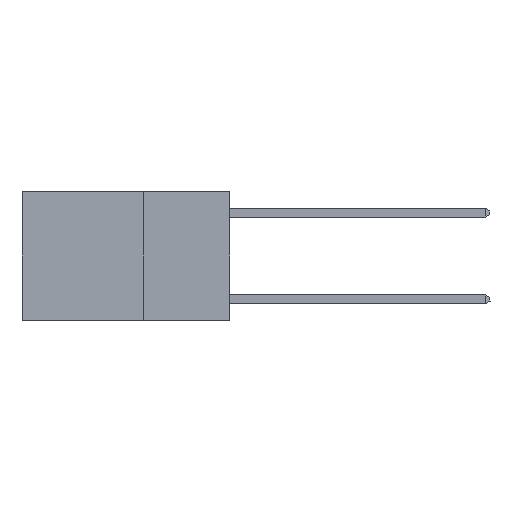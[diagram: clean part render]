
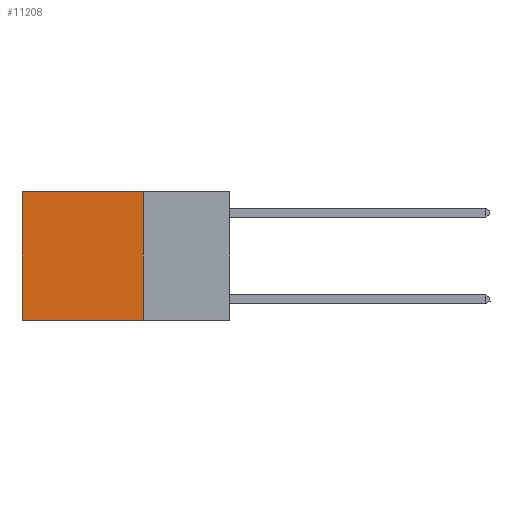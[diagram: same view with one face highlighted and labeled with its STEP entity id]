
A CAD part, left-side view. The second image highlights one B-rep face of the part: STEP entity #11208.
In plain terms, the highlighted planar face has unit normal (-1, 0, 0).
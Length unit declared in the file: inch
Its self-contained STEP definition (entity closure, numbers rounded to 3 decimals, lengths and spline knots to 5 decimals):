
#1647 = CARTESIAN_POINT ( 'NONE',  ( 0.2625, 0.25, -0.37 ) ) ;
#2229 = VECTOR ( 'NONE', #18958, 39.37008 ) ;
#3643 = EDGE_LOOP ( 'NONE', ( #12817, #16728, #27939, #23539 ) ) ;
#3807 = VECTOR ( 'NONE', #9278, 39.37008 ) ;
#4375 = VECTOR ( 'NONE', #17490, 39.37008 ) ;
#5471 = PLANE ( 'NONE',  #10500 ) ;
#6125 = LINE ( 'NONE', #1647, #4375 ) ;
#6558 = VERTEX_POINT ( 'NONE', #11032 ) ;
#6882 = CARTESIAN_POINT ( 'NONE',  ( 0.2625, 0.25, 0. ) ) ;
#6958 = LINE ( 'NONE', #11903, #3807 ) ;
#7930 = DIRECTION ( 'NONE',  ( 1., 0., 0. ) ) ;
#9261 = VERTEX_POINT ( 'NONE', #29301 ) ;
#9278 = DIRECTION ( 'NONE',  ( 0., 0., -1. ) ) ;
#10500 = AXIS2_PLACEMENT_3D ( 'NONE', #28296, #7930, #23500 ) ;
#11032 = CARTESIAN_POINT ( 'NONE',  ( 0.2625, 0.6, 0. ) ) ;
#11208 = ADVANCED_FACE ( 'NONE', ( #14159 ), #5471, .F. ) ;
#11903 = CARTESIAN_POINT ( 'NONE',  ( 0.2625, 0.25, 0. ) ) ;
#12817 = ORIENTED_EDGE ( 'NONE', *, *, #23487, .T. ) ;
#12876 = LINE ( 'NONE', #24923, #15382 ) ;
#14159 = FACE_OUTER_BOUND ( 'NONE', #3643, .T. ) ;
#14876 = EDGE_CURVE ( 'NONE', #22967, #9261, #6125, .T. ) ;
#15382 = VECTOR ( 'NONE', #20441, 39.37008 ) ;
#16728 = ORIENTED_EDGE ( 'NONE', *, *, #14876, .F. ) ;
#16748 = CARTESIAN_POINT ( 'NONE',  ( 0.2625, 0.25, 0. ) ) ;
#17490 = DIRECTION ( 'NONE',  ( 0., 1., 0. ) ) ;
#18958 = DIRECTION ( 'NONE',  ( 0., 1., 0. ) ) ;
#19355 = LINE ( 'NONE', #16748, #2229 ) ;
#20441 = DIRECTION ( 'NONE',  ( 0., 0., -1. ) ) ;
#20836 = EDGE_CURVE ( 'NONE', #22636, #22967, #6958, .T. ) ;
#22636 = VERTEX_POINT ( 'NONE', #6882 ) ;
#22862 = EDGE_CURVE ( 'NONE', #22636, #6558, #19355, .T. ) ;
#22967 = VERTEX_POINT ( 'NONE', #25508 ) ;
#23487 = EDGE_CURVE ( 'NONE', #6558, #9261, #12876, .T. ) ;
#23500 = DIRECTION ( 'NONE',  ( 0., 0., -1. ) ) ;
#23539 = ORIENTED_EDGE ( 'NONE', *, *, #22862, .T. ) ;
#24923 = CARTESIAN_POINT ( 'NONE',  ( 0.2625, 0.6, 0. ) ) ;
#25508 = CARTESIAN_POINT ( 'NONE',  ( 0.2625, 0.25, -0.37 ) ) ;
#27939 = ORIENTED_EDGE ( 'NONE', *, *, #20836, .F. ) ;
#28296 = CARTESIAN_POINT ( 'NONE',  ( 0.2625, 0.25, 0. ) ) ;
#29301 = CARTESIAN_POINT ( 'NONE',  ( 0.2625, 0.6, -0.37 ) ) ;
